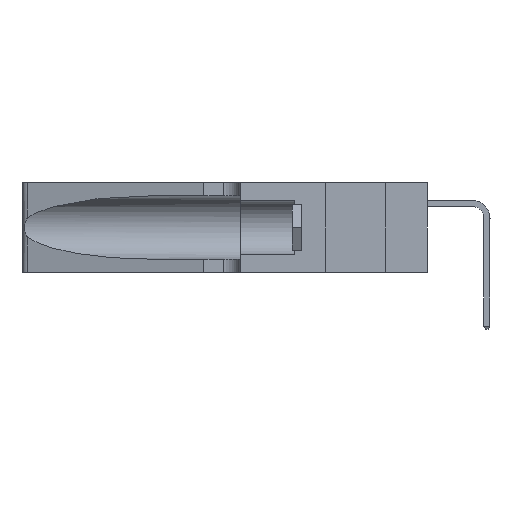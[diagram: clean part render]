
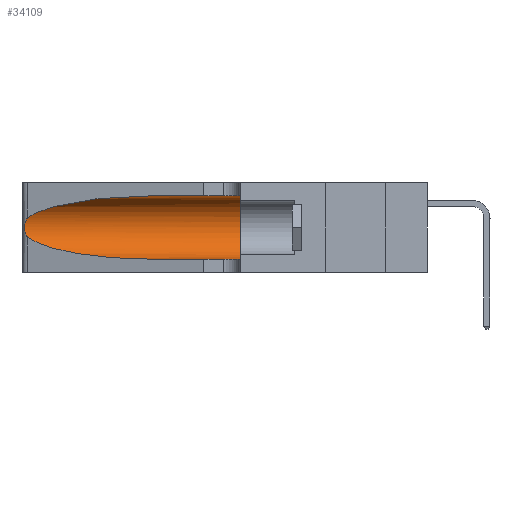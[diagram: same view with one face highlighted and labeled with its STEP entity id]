
A CAD part, left-side view. The second image highlights one B-rep face of the part: STEP entity #34109.
In plain terms, the highlighted cylindrical face has radius 3.308 mm (diameter 6.617 mm), a partial arc.
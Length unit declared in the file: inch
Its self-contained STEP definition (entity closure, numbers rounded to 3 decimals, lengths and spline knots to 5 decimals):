
#125 = CARTESIAN_POINT ( 'NONE',  ( 0.1305, 0.72297, 0.31525 ) ) ;
#520 = ORIENTED_EDGE ( 'NONE', *, *, #27695, .F. ) ;
#586 = EDGE_CURVE ( 'NONE', #41907, #46853, #5767, .T. ) ;
#985 = CARTESIAN_POINT ( 'NONE',  ( 0.1305, 0.72297, 0.05475 ) ) ;
#1557 = DIRECTION ( 'NONE',  ( 0., -1., 0. ) ) ;
#2993 = CARTESIAN_POINT ( 'NONE',  ( 0.1305, 0.35, 0.185 ) ) ;
#3470 = CARTESIAN_POINT ( 'NONE',  ( 0.26075, 1.23896, 0.178 ) ) ;
#4091 = CARTESIAN_POINT ( 'NONE',  ( 0.25487, 1.22718, 0.22369 ) ) ;
#4867 = VERTEX_POINT ( 'NONE', #33088 ) ;
#5767 = LINE ( 'NONE', #20312, #44708 ) ;
#6769 = DIRECTION ( 'NONE',  ( 0., 0., 1. ) ) ;
#7234 = CARTESIAN_POINT ( 'NONE',  ( 0.25856, 1.23593, 0.16098 ) ) ;
#8572 = LINE ( 'NONE', #34100, #28635 ) ;
#8638 = CARTESIAN_POINT ( 'NONE',  ( 0.25487, 1.22718, 0.14631 ) ) ;
#10867 = CARTESIAN_POINT ( 'NONE',  ( 0.25639, 1.23184, 0.21858 ) ) ;
#11028 = CARTESIAN_POINT ( 'NONE',  ( 0.25639, 1.23186, 0.15144 ) ) ;
#13987 = ORIENTED_EDGE ( 'NONE', *, *, #22934, .T. ) ;
#14810 = CARTESIAN_POINT ( 'NONE',  ( 0.25487, 1.22718, 0.14631 ) ) ;
#15295 = DIRECTION ( 'NONE',  ( 0., -1., 0. ) ) ;
#15534 = FACE_OUTER_BOUND ( 'NONE', #16819, .T. ) ;
#15958 = CARTESIAN_POINT ( 'NONE',  ( 0.2373, 1.15595, 0.08982 ) ) ;
#16819 = EDGE_LOOP ( 'NONE', ( #20466, #13987, #17526, #25828, #520, #40599 ) ) ;
#17199 = CARTESIAN_POINT ( 'NONE',  ( 0.2373, 1.15595, 0.28018 ) ) ;
#17526 = ORIENTED_EDGE ( 'NONE', *, *, #36070, .T. ) ;
#18423 = CARTESIAN_POINT ( 'NONE',  ( 0.25487, 1.22718, 0.22369 ) ) ;
#18887 = B_SPLINE_CURVE_WITH_KNOTS ( 'NONE', 3,
 ( #18423, #41029, #10867, #44828, #22234, #48615, #26015, #3470, #29833, #7234, #33628, #11028, #37405, #14810 ),
 .UNSPECIFIED., .F., .F.,
 ( 4, 2, 2, 2, 2, 2, 4 ),
 ( 0., 0.00027, 0.00053, 0.00107, 0.0016, 0.00187, 0.00214 ),
 .UNSPECIFIED. ) ;
#19237 = DIRECTION ( 'NONE',  ( 0., -1., 0. ) ) ;
#20312 = CARTESIAN_POINT ( 'NONE',  ( 0.1305, 1.61858, 0.31525 ) ) ;
#20466 = ORIENTED_EDGE ( 'NONE', *, *, #26908, .T. ) ;
#22234 = CARTESIAN_POINT ( 'NONE',  ( 0.25854, 1.2359, 0.20912 ) ) ;
#22465 = AXIS2_PLACEMENT_3D ( 'NONE', #2993, #29363, #6769 ) ;
#22934 = EDGE_CURVE ( 'NONE', #29694, #34795, #18887, .T. ) ;
#23542 = CARTESIAN_POINT ( 'NONE',  ( 0.18966, 0.96281, 0.05475 ) ) ;
#25828 = ORIENTED_EDGE ( 'NONE', *, *, #27309, .T. ) ;
#26015 = CARTESIAN_POINT ( 'NONE',  ( 0.26075, 1.23896, 0.19203 ) ) ;
#26908 = EDGE_CURVE ( 'NONE', #41907, #29694, #36202, .T. ) ;
#27309 = EDGE_CURVE ( 'NONE', #33304, #4867, #8572, .T. ) ;
#27695 = EDGE_CURVE ( 'NONE', #46853, #4867, #38854, .T. ) ;
#28635 = VECTOR ( 'NONE', #15295, 39.37008 ) ;
#29363 = DIRECTION ( 'NONE',  ( 0., 1., 0. ) ) ;
#29631 =( BOUNDED_CURVE ( )  B_SPLINE_CURVE ( 3, ( #42337, #15958, #23542, #985 ),
 .UNSPECIFIED., .F., .T. ) 
 B_SPLINE_CURVE_WITH_KNOTS ( ( 4, 4 ),
 ( 3.44316, 4.71239 ),
 .UNSPECIFIED. ) 
 CURVE ( )  GEOMETRIC_REPRESENTATION_ITEM ( )  RATIONAL_B_SPLINE_CURVE ( ( 1., 0.87, 0.87, 1. ) ) 
 REPRESENTATION_ITEM ( '' )  );
#29694 = VERTEX_POINT ( 'NONE', #4091 ) ;
#29833 = CARTESIAN_POINT ( 'NONE',  ( 0.26017, 1.23833, 0.17102 ) ) ;
#32215 = CARTESIAN_POINT ( 'NONE',  ( 0.1305, 0.72297, 0.31525 ) ) ;
#33088 = CARTESIAN_POINT ( 'NONE',  ( 0.1305, 0.35, 0.05475 ) ) ;
#33304 = VERTEX_POINT ( 'NONE', #33880 ) ;
#33628 = CARTESIAN_POINT ( 'NONE',  ( 0.25789, 1.23486, 0.15765 ) ) ;
#33880 = CARTESIAN_POINT ( 'NONE',  ( 0.1305, 0.72297, 0.05475 ) ) ;
#34052 = CARTESIAN_POINT ( 'NONE',  ( 0.1305, 0.35, 0.31525 ) ) ;
#34100 = CARTESIAN_POINT ( 'NONE',  ( 0.1305, 1.61858, 0.05475 ) ) ;
#34109 = ADVANCED_FACE ( 'NONE', ( #15534 ), #44454, .F. ) ;
#34795 = VERTEX_POINT ( 'NONE', #8638 ) ;
#35855 = CARTESIAN_POINT ( 'NONE',  ( 0.18966, 0.96281, 0.31525 ) ) ;
#36070 = EDGE_CURVE ( 'NONE', #34795, #33304, #29631, .T. ) ;
#36202 =( BOUNDED_CURVE ( )  B_SPLINE_CURVE ( 3, ( #32215, #35855, #17199, #43596 ),
 .UNSPECIFIED., .F., .F. ) 
 B_SPLINE_CURVE_WITH_KNOTS ( ( 4, 4 ),
 ( 1.5708, 2.84003 ),
 .UNSPECIFIED. ) 
 CURVE ( )  GEOMETRIC_REPRESENTATION_ITEM ( )  RATIONAL_B_SPLINE_CURVE ( ( 1., 0.87, 0.87, 1. ) ) 
 REPRESENTATION_ITEM ( '' )  );
#37405 = CARTESIAN_POINT ( 'NONE',  ( 0.25555, 1.22993, 0.14849 ) ) ;
#37886 = CARTESIAN_POINT ( 'NONE',  ( 0.1305, 1.61858, 0.185 ) ) ;
#38854 = CIRCLE ( 'NONE', #22465, 0.13025 ) ;
#39991 = AXIS2_PLACEMENT_3D ( 'NONE', #37886, #19237, #41832 ) ;
#40599 = ORIENTED_EDGE ( 'NONE', *, *, #586, .F. ) ;
#41029 = CARTESIAN_POINT ( 'NONE',  ( 0.25555, 1.22994, 0.2215 ) ) ;
#41832 = DIRECTION ( 'NONE',  ( 0., 0., -1. ) ) ;
#41907 = VERTEX_POINT ( 'NONE', #125 ) ;
#42337 = CARTESIAN_POINT ( 'NONE',  ( 0.25487, 1.22718, 0.14631 ) ) ;
#43596 = CARTESIAN_POINT ( 'NONE',  ( 0.25487, 1.22718, 0.22369 ) ) ;
#44454 = CYLINDRICAL_SURFACE ( 'NONE', #39991, 0.13025 ) ;
#44708 = VECTOR ( 'NONE', #1557, 39.37008 ) ;
#44828 = CARTESIAN_POINT ( 'NONE',  ( 0.25787, 1.23484, 0.2124 ) ) ;
#46853 = VERTEX_POINT ( 'NONE', #34052 ) ;
#48615 = CARTESIAN_POINT ( 'NONE',  ( 0.26018, 1.23835, 0.19895 ) ) ;
